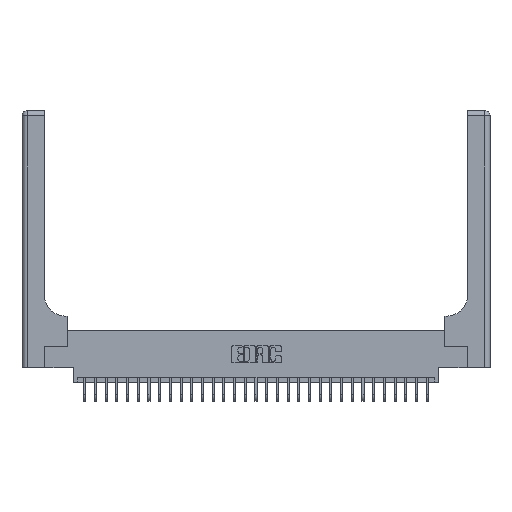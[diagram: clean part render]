
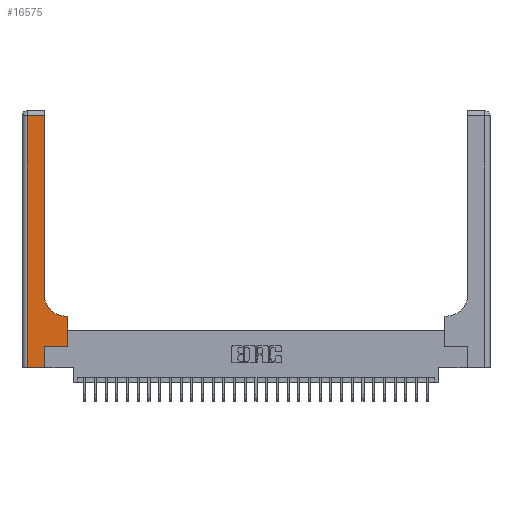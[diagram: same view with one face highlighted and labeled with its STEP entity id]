
A CAD part, top view. The second image highlights one B-rep face of the part: STEP entity #16575.
In plain terms, the highlighted planar face has unit normal (0, 0, 1).
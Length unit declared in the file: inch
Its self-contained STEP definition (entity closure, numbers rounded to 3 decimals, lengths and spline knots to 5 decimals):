
#1048 = CARTESIAN_POINT ( 'NONE',  ( 0.528, 0.25, 0.37 ) ) ;
#1076 = EDGE_CURVE ( 'NONE', #2272, #11060, #29834, .T. ) ;
#1094 = DIRECTION ( 'NONE',  ( 0., 0., -1. ) ) ;
#1165 = DIRECTION ( 'NONE',  ( 1., 0., 0. ) ) ;
#1185 = VECTOR ( 'NONE', #26122, 39.37008 ) ;
#1505 = VERTEX_POINT ( 'NONE', #13838 ) ;
#1642 = VECTOR ( 'NONE', #20397, 39.37008 ) ;
#2034 = LINE ( 'NONE', #21549, #21156 ) ;
#2149 = VERTEX_POINT ( 'NONE', #7002 ) ;
#2272 = VERTEX_POINT ( 'NONE', #25843 ) ;
#2685 = AXIS2_PLACEMENT_3D ( 'NONE', #25854, #12071, #14388 ) ;
#3026 = FACE_OUTER_BOUND ( 'NONE', #12919, .T. ) ;
#4922 = VECTOR ( 'NONE', #22963, 39.37008 ) ;
#5088 = PLANE ( 'NONE',  #2685 ) ;
#5474 = VERTEX_POINT ( 'NONE', #13110 ) ;
#5710 = ORIENTED_EDGE ( 'NONE', *, *, #1076, .T. ) ;
#5974 = ORIENTED_EDGE ( 'NONE', *, *, #14668, .T. ) ;
#6378 = CARTESIAN_POINT ( 'NONE',  ( 0.265, 0., 0.37 ) ) ;
#6719 = CARTESIAN_POINT ( 'NONE',  ( 0.528, 0.25, 0.37 ) ) ;
#7002 = CARTESIAN_POINT ( 'NONE',  ( 0.528, 0.6, 0.37 ) ) ;
#7412 = LINE ( 'NONE', #18149, #1642 ) ;
#7463 = ORIENTED_EDGE ( 'NONE', *, *, #10235, .T. ) ;
#8400 = LINE ( 'NONE', #18980, #10207 ) ;
#9820 = AXIS2_PLACEMENT_3D ( 'NONE', #26283, #1094, #14920 ) ;
#10207 = VECTOR ( 'NONE', #16597, 39.37008 ) ;
#10235 = EDGE_CURVE ( 'NONE', #26977, #15818, #2034, .T. ) ;
#10254 = ORIENTED_EDGE ( 'NONE', *, *, #22238, .T. ) ;
#11060 = VERTEX_POINT ( 'NONE', #6378 ) ;
#12071 = DIRECTION ( 'NONE',  ( 0., 0., -1. ) ) ;
#12184 = ORIENTED_EDGE ( 'NONE', *, *, #13190, .T. ) ;
#12207 = CARTESIAN_POINT ( 'NONE',  ( 0.26, 0.85, 0.37 ) ) ;
#12270 = DIRECTION ( 'NONE',  ( 0., -1., 0. ) ) ;
#12673 = LINE ( 'NONE', #25941, #24223 ) ;
#12919 = EDGE_LOOP ( 'NONE', ( #18621, #12184, #18386, #5710, #22394, #7463, #27991, #10254, #5974 ) ) ;
#13110 = CARTESIAN_POINT ( 'NONE',  ( 0.51, 0.6, 0.37 ) ) ;
#13190 = EDGE_CURVE ( 'NONE', #28086, #1505, #8400, .T. ) ;
#13838 = CARTESIAN_POINT ( 'NONE',  ( 0.06, 2.94, 0.37 ) ) ;
#14317 = EDGE_CURVE ( 'NONE', #21432, #28086, #18651, .T. ) ;
#14388 = DIRECTION ( 'NONE',  ( -1., 0., 0. ) ) ;
#14668 = EDGE_CURVE ( 'NONE', #5474, #21432, #26221, .T. ) ;
#14909 = DIRECTION ( 'NONE',  ( 1., 0., 0. ) ) ;
#14920 = DIRECTION ( 'NONE',  ( 1., 0., 0. ) ) ;
#15818 = VERTEX_POINT ( 'NONE', #1048 ) ;
#16490 = VECTOR ( 'NONE', #1165, 39.37008 ) ;
#16575 = ADVANCED_FACE ( 'NONE', ( #3026 ), #5088, .F. ) ;
#16597 = DIRECTION ( 'NONE',  ( -1., 0., 0. ) ) ;
#17234 = EDGE_CURVE ( 'NONE', #11060, #26977, #26081, .T. ) ;
#18149 = CARTESIAN_POINT ( 'NONE',  ( 0.26, 0.6, 0.37 ) ) ;
#18386 = ORIENTED_EDGE ( 'NONE', *, *, #28290, .T. ) ;
#18610 = LINE ( 'NONE', #6719, #4922 ) ;
#18621 = ORIENTED_EDGE ( 'NONE', *, *, #14317, .T. ) ;
#18651 = LINE ( 'NONE', #26896, #23050 ) ;
#18980 = CARTESIAN_POINT ( 'NONE',  ( 0., 2.94, 0.37 ) ) ;
#20397 = DIRECTION ( 'NONE',  ( -1., 0., 0. ) ) ;
#21156 = VECTOR ( 'NONE', #14909, 39.37008 ) ;
#21432 = VERTEX_POINT ( 'NONE', #12207 ) ;
#21549 = CARTESIAN_POINT ( 'NONE',  ( 0.265, 0.25, 0.37 ) ) ;
#21683 = CARTESIAN_POINT ( 'NONE',  ( 0.265, 0.25, 0.37 ) ) ;
#21787 = EDGE_CURVE ( 'NONE', #15818, #2149, #18610, .T. ) ;
#22238 = EDGE_CURVE ( 'NONE', #2149, #5474, #7412, .T. ) ;
#22394 = ORIENTED_EDGE ( 'NONE', *, *, #17234, .T. ) ;
#22963 = DIRECTION ( 'NONE',  ( 0., 1., 0. ) ) ;
#23050 = VECTOR ( 'NONE', #29066, 39.37008 ) ;
#23255 = CARTESIAN_POINT ( 'NONE',  ( 0.26, 2.94, 0.37 ) ) ;
#23854 = CARTESIAN_POINT ( 'NONE',  ( 0.265, 0., 0.37 ) ) ;
#24223 = VECTOR ( 'NONE', #12270, 39.37008 ) ;
#25843 = CARTESIAN_POINT ( 'NONE',  ( 0.06, 0., 0.37 ) ) ;
#25854 = CARTESIAN_POINT ( 'NONE',  ( 0., 3., 0.37 ) ) ;
#25941 = CARTESIAN_POINT ( 'NONE',  ( 0.06, 3., 0.37 ) ) ;
#26081 = LINE ( 'NONE', #23854, #1185 ) ;
#26122 = DIRECTION ( 'NONE',  ( 0., 1., 0. ) ) ;
#26221 = CIRCLE ( 'NONE', #9820, 0.25 ) ;
#26283 = CARTESIAN_POINT ( 'NONE',  ( 0.51, 0.85, 0.37 ) ) ;
#26896 = CARTESIAN_POINT ( 'NONE',  ( 0.26, 3., 0.37 ) ) ;
#26977 = VERTEX_POINT ( 'NONE', #21683 ) ;
#27991 = ORIENTED_EDGE ( 'NONE', *, *, #21787, .T. ) ;
#28086 = VERTEX_POINT ( 'NONE', #23255 ) ;
#28290 = EDGE_CURVE ( 'NONE', #1505, #2272, #12673, .T. ) ;
#28702 = CARTESIAN_POINT ( 'NONE',  ( 0., 0., 0.37 ) ) ;
#29066 = DIRECTION ( 'NONE',  ( 0., 1., 0. ) ) ;
#29834 = LINE ( 'NONE', #28702, #16490 ) ;
